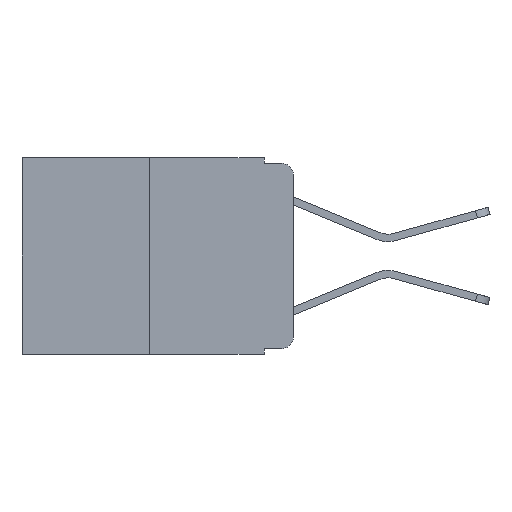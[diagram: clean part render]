
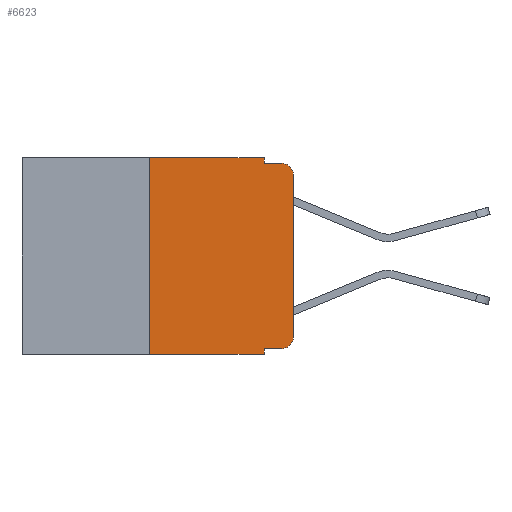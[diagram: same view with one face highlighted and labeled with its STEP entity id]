
A CAD part, left-side view. The second image highlights one B-rep face of the part: STEP entity #6623.
In plain terms, the highlighted planar face has unit normal (-1, 0, 0).
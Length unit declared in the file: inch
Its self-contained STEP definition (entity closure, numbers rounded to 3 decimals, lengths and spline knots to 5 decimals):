
#185 = ORIENTED_EDGE ( 'NONE', *, *, #19759, .T. ) ;
#415 = CARTESIAN_POINT ( 'NONE',  ( 0., 0.473, 0. ) ) ;
#521 = DIRECTION ( 'NONE',  ( 0., 0., 1. ) ) ;
#815 = EDGE_LOOP ( 'NONE', ( #19620, #11544, #18115, #16307, #2134, #1468, #10000, #7802, #185, #22281 ) ) ;
#874 = CARTESIAN_POINT ( 'NONE',  ( 0., 0.051, -0.333 ) ) ;
#1220 = CARTESIAN_POINT ( 'NONE',  ( 0., 0.051, 0. ) ) ;
#1468 = ORIENTED_EDGE ( 'NONE', *, *, #7118, .F. ) ;
#2134 = ORIENTED_EDGE ( 'NONE', *, *, #15477, .F. ) ;
#2257 = LINE ( 'NONE', #6529, #12377 ) ;
#2485 = DIRECTION ( 'NONE',  ( 0., -1., 0. ) ) ;
#2723 = VERTEX_POINT ( 'NONE', #22619 ) ;
#3057 = CARTESIAN_POINT ( 'NONE',  ( 0., 0.473, 0. ) ) ;
#3147 = DIRECTION ( 'NONE',  ( 0., 0., -1. ) ) ;
#3202 = CARTESIAN_POINT ( 'NONE',  ( 0., 0.02, -0.01 ) ) ;
#3642 = VERTEX_POINT ( 'NONE', #3202 ) ;
#3770 = CARTESIAN_POINT ( 'NONE',  ( 0., 0.051, 0. ) ) ;
#3818 = CARTESIAN_POINT ( 'NONE',  ( 0., 0.473, -0.343 ) ) ;
#4209 = DIRECTION ( 'NONE',  ( -1., 0., 0. ) ) ;
#4684 = CARTESIAN_POINT ( 'NONE',  ( 0., 0.02, -0.333 ) ) ;
#5043 = VECTOR ( 'NONE', #20931, 39.37008 ) ;
#5232 = VECTOR ( 'NONE', #2485, 39.37008 ) ;
#5438 = VECTOR ( 'NONE', #25761, 39.37008 ) ;
#5547 = CIRCLE ( 'NONE', #18504, 0.02 ) ;
#6054 = LINE ( 'NONE', #3818, #5438 ) ;
#6529 = CARTESIAN_POINT ( 'NONE',  ( 0., 0.051, 0. ) ) ;
#6623 = ADVANCED_FACE ( 'NONE', ( #16047 ), #13231, .F. ) ;
#7118 = EDGE_CURVE ( 'NONE', #13287, #2723, #25925, .T. ) ;
#7441 = VERTEX_POINT ( 'NONE', #1220 ) ;
#7630 = EDGE_CURVE ( 'NONE', #14716, #16298, #24050, .T. ) ;
#7802 = ORIENTED_EDGE ( 'NONE', *, *, #7630, .F. ) ;
#7831 = DIRECTION ( 'NONE',  ( 0., 0., -1. ) ) ;
#7929 = VECTOR ( 'NONE', #16842, 39.37008 ) ;
#9530 = CARTESIAN_POINT ( 'NONE',  ( 0., 0.051, -0.343 ) ) ;
#10000 = ORIENTED_EDGE ( 'NONE', *, *, #10863, .T. ) ;
#10863 = EDGE_CURVE ( 'NONE', #13287, #16298, #6054, .T. ) ;
#11042 = VERTEX_POINT ( 'NONE', #14417 ) ;
#11190 = EDGE_CURVE ( 'NONE', #11042, #3642, #19268, .T. ) ;
#11544 = ORIENTED_EDGE ( 'NONE', *, *, #15245, .T. ) ;
#11953 = CARTESIAN_POINT ( 'NONE',  ( 0., 0.02, -0.03 ) ) ;
#12377 = VECTOR ( 'NONE', #16561, 39.37008 ) ;
#12516 = VERTEX_POINT ( 'NONE', #19164 ) ;
#12730 = CARTESIAN_POINT ( 'NONE',  ( 0., 0.25, 0. ) ) ;
#13062 = CARTESIAN_POINT ( 'NONE',  ( 0., 0.25, -0.343 ) ) ;
#13231 = PLANE ( 'NONE',  #20028 ) ;
#13287 = VERTEX_POINT ( 'NONE', #13062 ) ;
#13350 = CIRCLE ( 'NONE', #21335, 0.02 ) ;
#13502 = VECTOR ( 'NONE', #7831, 39.37008 ) ;
#13984 = DIRECTION ( 'NONE',  ( 0., 0., -1. ) ) ;
#14201 = CARTESIAN_POINT ( 'NONE',  ( 0., 0.051, -0.333 ) ) ;
#14328 = CARTESIAN_POINT ( 'NONE',  ( 0., 0., -0.313 ) ) ;
#14417 = CARTESIAN_POINT ( 'NONE',  ( 0., 0.051, -0.01 ) ) ;
#14716 = VERTEX_POINT ( 'NONE', #14201 ) ;
#15208 = LINE ( 'NONE', #21320, #25103 ) ;
#15243 = DIRECTION ( 'NONE',  ( 1., 0., 0. ) ) ;
#15245 = EDGE_CURVE ( 'NONE', #12516, #3642, #5547, .T. ) ;
#15477 = EDGE_CURVE ( 'NONE', #2723, #7441, #16553, .T. ) ;
#16047 = FACE_OUTER_BOUND ( 'NONE', #815, .T. ) ;
#16275 = CARTESIAN_POINT ( 'NONE',  ( 0., 0.02, -0.313 ) ) ;
#16298 = VERTEX_POINT ( 'NONE', #9530 ) ;
#16307 = ORIENTED_EDGE ( 'NONE', *, *, #23696, .F. ) ;
#16553 = LINE ( 'NONE', #415, #5232 ) ;
#16561 = DIRECTION ( 'NONE',  ( 0., 0., -1. ) ) ;
#16842 = DIRECTION ( 'NONE',  ( 0., -1., 0. ) ) ;
#17216 = VERTEX_POINT ( 'NONE', #14328 ) ;
#18115 = ORIENTED_EDGE ( 'NONE', *, *, #11190, .F. ) ;
#18288 = DIRECTION ( 'NONE',  ( 0., 0., -1. ) ) ;
#18504 = AXIS2_PLACEMENT_3D ( 'NONE', #11953, #25843, #13984 ) ;
#18767 = CARTESIAN_POINT ( 'NONE',  ( 0., 0.051, -0.01 ) ) ;
#19164 = CARTESIAN_POINT ( 'NONE',  ( 0., 0., -0.03 ) ) ;
#19268 = LINE ( 'NONE', #18767, #7929 ) ;
#19620 = ORIENTED_EDGE ( 'NONE', *, *, #24515, .T. ) ;
#19759 = EDGE_CURVE ( 'NONE', #14716, #23742, #25654, .T. ) ;
#20028 = AXIS2_PLACEMENT_3D ( 'NONE', #3057, #15243, #3147 ) ;
#20931 = DIRECTION ( 'NONE',  ( 0., -1., 0. ) ) ;
#21320 = CARTESIAN_POINT ( 'NONE',  ( 0., 0., 0. ) ) ;
#21335 = AXIS2_PLACEMENT_3D ( 'NONE', #16275, #4209, #18288 ) ;
#22281 = ORIENTED_EDGE ( 'NONE', *, *, #24178, .T. ) ;
#22619 = CARTESIAN_POINT ( 'NONE',  ( 0., 0.25, 0. ) ) ;
#23291 = DIRECTION ( 'NONE',  ( 0., 0., 1. ) ) ;
#23696 = EDGE_CURVE ( 'NONE', #7441, #11042, #2257, .T. ) ;
#23742 = VERTEX_POINT ( 'NONE', #4684 ) ;
#24050 = LINE ( 'NONE', #3770, #13502 ) ;
#24178 = EDGE_CURVE ( 'NONE', #23742, #17216, #13350, .T. ) ;
#24515 = EDGE_CURVE ( 'NONE', #17216, #12516, #15208, .T. ) ;
#25103 = VECTOR ( 'NONE', #23291, 39.37008 ) ;
#25317 = VECTOR ( 'NONE', #521, 39.37008 ) ;
#25654 = LINE ( 'NONE', #874, #5043 ) ;
#25761 = DIRECTION ( 'NONE',  ( 0., -1., 0. ) ) ;
#25843 = DIRECTION ( 'NONE',  ( -1., 0., 0. ) ) ;
#25925 = LINE ( 'NONE', #12730, #25317 ) ;
